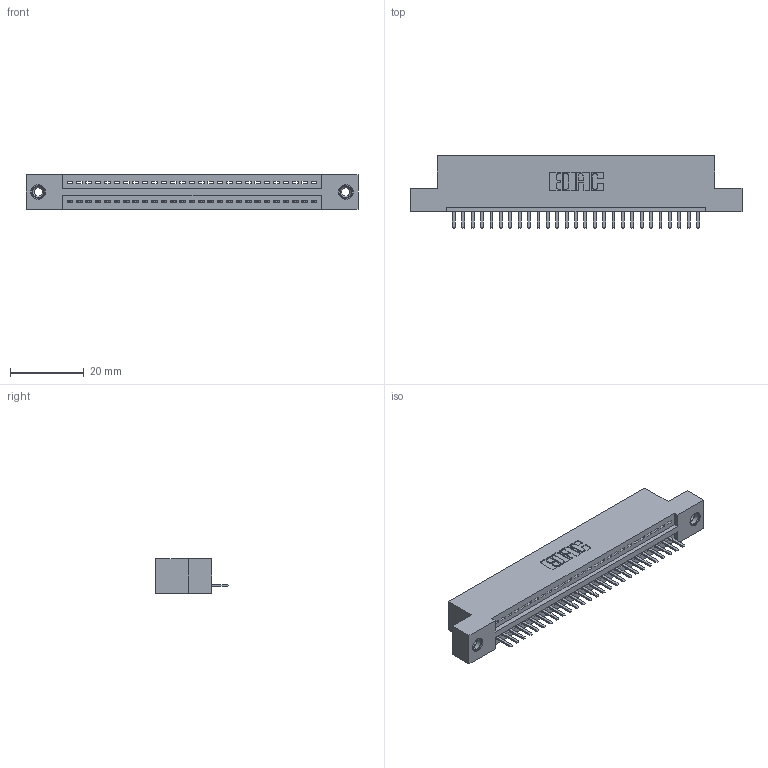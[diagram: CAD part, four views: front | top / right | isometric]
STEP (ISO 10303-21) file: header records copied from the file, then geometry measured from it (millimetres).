
FILE_DESCRIPTION (( 'STEP AP203' ), '1' );
FILE_NAME ('345-027-520-108.STEP', '2018-08-22T04:46:38', ( '' ), ( '' ), 'SwSTEP 2.0', 'SolidWorks 2016', '' );
FILE_SCHEMA (( 'CONFIG_CONTROL_DESIGN' ));
Length unit declared in the file: inch
Products named in the file (4): 345-250-001_345-250-003-102; 345-027-520-108; 345 Part_Flush Mounting Lugs - 0.156 Dia-TI; 345-292-001_345-293-120
Assembly tree (30 placements, depth 2):
  345-027-520-108
    345 Part_Flush Mounting Lugs - 0.156 Dia-TI
    345-292-001_345-293-120  x27
    345-250-001_345-250-003-102  x2
Bounding box: 89.79 x 19.68 x 9.4 mm (x, y, z)
Volume: 8321.2 mm3; surface area: 10619.3 mm2
Topology: 30 solids, 30 shells, 1860 faces, 5445 edges, 3550 vertices
Faces by surface type: plane 1246, cylinder 598, cone 12, torus 4
Entity records: 23640 total; most frequent: CARTESIAN_POINT 4088, ORIENTED_EDGE 4030, DIRECTION 3607, EDGE_CURVE 2015, VECTOR 1751, LINE 1751, VERTEX_POINT 1336, AXIS2_PLACEMENT_3D 928
